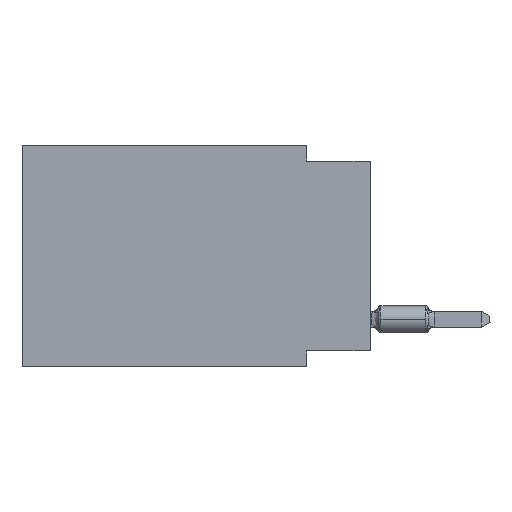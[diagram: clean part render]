
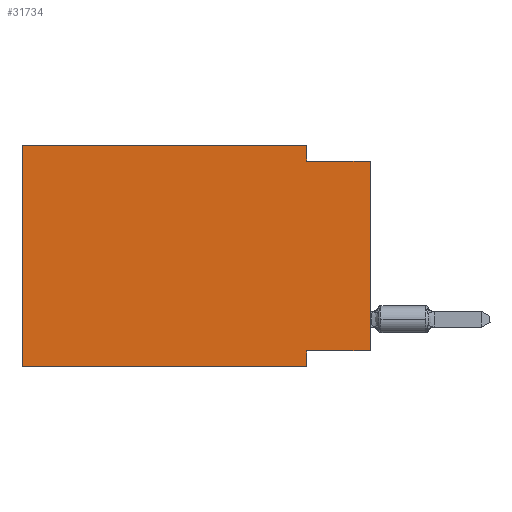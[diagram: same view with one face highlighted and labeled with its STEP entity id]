
A CAD part, left-side view. The second image highlights one B-rep face of the part: STEP entity #31734.
In plain terms, the highlighted planar face has unit normal (-1, 0, 0).
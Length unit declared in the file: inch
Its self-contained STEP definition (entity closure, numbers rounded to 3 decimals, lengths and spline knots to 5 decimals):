
#1047 = ORIENTED_EDGE ( 'NONE', *, *, #12733, .F. ) ;
#1056 = CARTESIAN_POINT ( 'NONE',  ( 0., 0.1, -0.025 ) ) ;
#1574 = EDGE_CURVE ( 'NONE', #32587, #12887, #9853, .T. ) ;
#2404 = CARTESIAN_POINT ( 'NONE',  ( 0., 0.1, -0.35 ) ) ;
#3716 = LINE ( 'NONE', #13909, #5486 ) ;
#3826 = ORIENTED_EDGE ( 'NONE', *, *, #25931, .T. ) ;
#4449 = EDGE_CURVE ( 'NONE', #23403, #19016, #6664, .T. ) ;
#4744 = CARTESIAN_POINT ( 'NONE',  ( 0., 0., -0.325 ) ) ;
#5126 = PLANE ( 'NONE',  #23129 ) ;
#5475 = EDGE_CURVE ( 'NONE', #12887, #19082, #30994, .T. ) ;
#5486 = VECTOR ( 'NONE', #29330, 39.37008 ) ;
#5793 = CARTESIAN_POINT ( 'NONE',  ( 0., 0.1, -0.325 ) ) ;
#6664 = LINE ( 'NONE', #25145, #11242 ) ;
#7825 = VECTOR ( 'NONE', #9691, 39.37008 ) ;
#8837 = CARTESIAN_POINT ( 'NONE',  ( 0., 0., -0.025 ) ) ;
#9134 = CARTESIAN_POINT ( 'NONE',  ( 0., 0.55, -0.35 ) ) ;
#9287 = EDGE_CURVE ( 'NONE', #23403, #25742, #19747, .T. ) ;
#9599 = CARTESIAN_POINT ( 'NONE',  ( 0., 0.55, 0. ) ) ;
#9691 = DIRECTION ( 'NONE',  ( 0., 0., -1. ) ) ;
#9853 = LINE ( 'NONE', #23089, #7825 ) ;
#11242 = VECTOR ( 'NONE', #22442, 39.37008 ) ;
#11297 = LINE ( 'NONE', #29919, #21822 ) ;
#11400 = EDGE_LOOP ( 'NONE', ( #3826, #15040, #16493, #22469, #26192, #32182, #31635, #1047 ) ) ;
#11958 = CARTESIAN_POINT ( 'NONE',  ( 0., 0.55, 0. ) ) ;
#12149 = EDGE_CURVE ( 'NONE', #14366, #19016, #3716, .T. ) ;
#12733 = EDGE_CURVE ( 'NONE', #13040, #14366, #28196, .T. ) ;
#12887 = VERTEX_POINT ( 'NONE', #1056 ) ;
#13040 = VERTEX_POINT ( 'NONE', #4744 ) ;
#13541 = DIRECTION ( 'NONE',  ( 0., -1., 0. ) ) ;
#13663 = VECTOR ( 'NONE', #14818, 39.37008 ) ;
#13909 = CARTESIAN_POINT ( 'NONE',  ( 0., 0.1, -0.35 ) ) ;
#14366 = VERTEX_POINT ( 'NONE', #5793 ) ;
#14818 = DIRECTION ( 'NONE',  ( 0., 1., 0. ) ) ;
#15040 = ORIENTED_EDGE ( 'NONE', *, *, #5475, .F. ) ;
#15497 = CARTESIAN_POINT ( 'NONE',  ( 0., 0.55, 0. ) ) ;
#16493 = ORIENTED_EDGE ( 'NONE', *, *, #1574, .F. ) ;
#17527 = CARTESIAN_POINT ( 'NONE',  ( 0., 0., -0.325 ) ) ;
#18462 = CARTESIAN_POINT ( 'NONE',  ( 0., 0., -0.025 ) ) ;
#19016 = VERTEX_POINT ( 'NONE', #2404 ) ;
#19082 = VERTEX_POINT ( 'NONE', #8837 ) ;
#19274 = EDGE_CURVE ( 'NONE', #25742, #32587, #24931, .T. ) ;
#19747 = LINE ( 'NONE', #11958, #30813 ) ;
#20028 = CARTESIAN_POINT ( 'NONE',  ( 0., 0.55, 0. ) ) ;
#21084 = DIRECTION ( 'NONE',  ( 0., 0., -1. ) ) ;
#21822 = VECTOR ( 'NONE', #27051, 39.37008 ) ;
#22442 = DIRECTION ( 'NONE',  ( 0., -1., 0. ) ) ;
#22448 = CARTESIAN_POINT ( 'NONE',  ( 0., 0.1, 0. ) ) ;
#22469 = ORIENTED_EDGE ( 'NONE', *, *, #19274, .F. ) ;
#23089 = CARTESIAN_POINT ( 'NONE',  ( 0., 0.1, 0. ) ) ;
#23129 = AXIS2_PLACEMENT_3D ( 'NONE', #15497, #31419, #21084 ) ;
#23403 = VERTEX_POINT ( 'NONE', #9134 ) ;
#23734 = VECTOR ( 'NONE', #30352, 39.37008 ) ;
#24931 = LINE ( 'NONE', #20028, #23734 ) ;
#25145 = CARTESIAN_POINT ( 'NONE',  ( 0., 0.55, -0.35 ) ) ;
#25742 = VERTEX_POINT ( 'NONE', #9599 ) ;
#25931 = EDGE_CURVE ( 'NONE', #13040, #19082, #11297, .T. ) ;
#26192 = ORIENTED_EDGE ( 'NONE', *, *, #9287, .F. ) ;
#27051 = DIRECTION ( 'NONE',  ( 0., 0., 1. ) ) ;
#28196 = LINE ( 'NONE', #17527, #13663 ) ;
#28372 = FACE_OUTER_BOUND ( 'NONE', #11400, .T. ) ;
#29330 = DIRECTION ( 'NONE',  ( 0., 0., -1. ) ) ;
#29919 = CARTESIAN_POINT ( 'NONE',  ( 0., 0., 0. ) ) ;
#30220 = VECTOR ( 'NONE', #13541, 39.37008 ) ;
#30352 = DIRECTION ( 'NONE',  ( 0., -1., 0. ) ) ;
#30424 = DIRECTION ( 'NONE',  ( 0., 0., 1. ) ) ;
#30813 = VECTOR ( 'NONE', #30424, 39.37008 ) ;
#30994 = LINE ( 'NONE', #18462, #30220 ) ;
#31419 = DIRECTION ( 'NONE',  ( 1., 0., 0. ) ) ;
#31635 = ORIENTED_EDGE ( 'NONE', *, *, #12149, .F. ) ;
#31734 = ADVANCED_FACE ( 'NONE', ( #28372 ), #5126, .F. ) ;
#32182 = ORIENTED_EDGE ( 'NONE', *, *, #4449, .T. ) ;
#32587 = VERTEX_POINT ( 'NONE', #22448 ) ;
